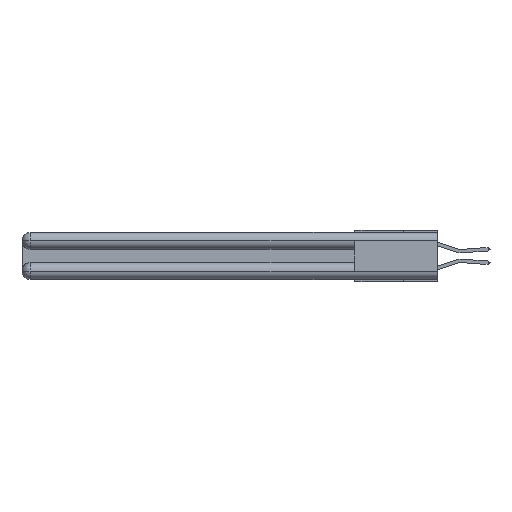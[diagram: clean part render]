
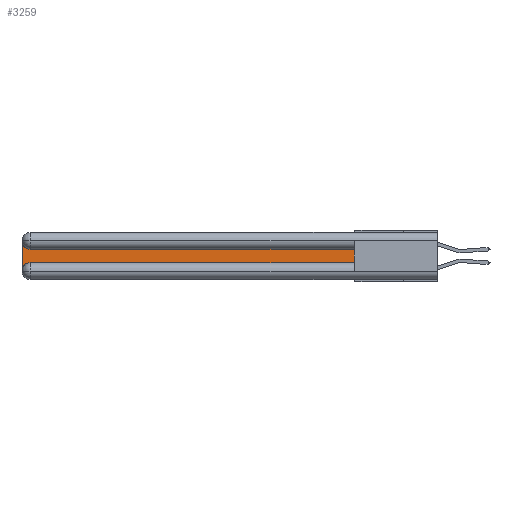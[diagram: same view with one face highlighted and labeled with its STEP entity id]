
A CAD part, left-side view. The second image highlights one B-rep face of the part: STEP entity #3259.
In plain terms, the highlighted planar face has unit normal (-1, 0, 0).
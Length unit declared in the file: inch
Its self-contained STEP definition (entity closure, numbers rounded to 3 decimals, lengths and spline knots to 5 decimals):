
#345 = CARTESIAN_POINT ( 'NONE',  ( 0.075, 2.94, -0.2775 ) ) ;
#422 = VECTOR ( 'NONE', #17137, 39.37008 ) ;
#693 = CARTESIAN_POINT ( 'NONE',  ( 0.075, 0.6, -0.1225 ) ) ;
#921 = AXIS2_PLACEMENT_3D ( 'NONE', #20512, #23227, #17745 ) ;
#1633 = CIRCLE ( 'NONE', #7621, 0.06 ) ;
#1658 = ORIENTED_EDGE ( 'NONE', *, *, #11270, .T. ) ;
#1872 = CARTESIAN_POINT ( 'NONE',  ( 0.075, 0.6, -0.1225 ) ) ;
#2462 = EDGE_CURVE ( 'NONE', #32187, #11492, #11005, .T. ) ;
#2471 = VERTEX_POINT ( 'NONE', #18239 ) ;
#2899 = DIRECTION ( 'NONE',  ( 1., 0., 0. ) ) ;
#3259 = ADVANCED_FACE ( 'NONE', ( #13729 ), #5594, .F. ) ;
#3362 = CARTESIAN_POINT ( 'NONE',  ( 0.075, 2.94, -0.2175 ) ) ;
#5594 = PLANE ( 'NONE',  #921 ) ;
#5992 = ORIENTED_EDGE ( 'NONE', *, *, #32218, .T. ) ;
#6529 = DIRECTION ( 'NONE',  ( 0., 0., -1. ) ) ;
#7053 = VECTOR ( 'NONE', #26360, 39.37008 ) ;
#7621 = AXIS2_PLACEMENT_3D ( 'NONE', #19111, #19005, #6529 ) ;
#8531 = CARTESIAN_POINT ( 'NONE',  ( 0.075, 3., -0.2775 ) ) ;
#8834 = ORIENTED_EDGE ( 'NONE', *, *, #2462, .T. ) ;
#9032 = EDGE_CURVE ( 'NONE', #11203, #17176, #18721, .T. ) ;
#9542 = CARTESIAN_POINT ( 'NONE',  ( 0.075, 0.6, -0.2175 ) ) ;
#10219 = ORIENTED_EDGE ( 'NONE', *, *, #11001, .T. ) ;
#11001 = EDGE_CURVE ( 'NONE', #17176, #32187, #1633, .T. ) ;
#11005 = LINE ( 'NONE', #31234, #12163 ) ;
#11203 = VERTEX_POINT ( 'NONE', #693 ) ;
#11270 = EDGE_CURVE ( 'NONE', #24827, #2471, #26851, .T. ) ;
#11492 = VERTEX_POINT ( 'NONE', #8531 ) ;
#12163 = VECTOR ( 'NONE', #16133, 39.37008 ) ;
#13073 = DIRECTION ( 'NONE',  ( 0., 0., -1. ) ) ;
#13291 = CARTESIAN_POINT ( 'NONE',  ( 0.075, 3., -0.0625 ) ) ;
#13729 = FACE_OUTER_BOUND ( 'NONE', #24518, .T. ) ;
#13787 = LINE ( 'NONE', #23938, #7053 ) ;
#14293 = CIRCLE ( 'NONE', #29495, 0.06 ) ;
#14594 = CARTESIAN_POINT ( 'NONE',  ( 0.075, 2.94, -0.1225 ) ) ;
#15156 = VECTOR ( 'NONE', #21952, 39.37008 ) ;
#16133 = DIRECTION ( 'NONE',  ( 0., 0., -1. ) ) ;
#17137 = DIRECTION ( 'NONE',  ( 0., -1., 0. ) ) ;
#17176 = VERTEX_POINT ( 'NONE', #14594 ) ;
#17745 = DIRECTION ( 'NONE',  ( 0., 0., -1. ) ) ;
#18239 = CARTESIAN_POINT ( 'NONE',  ( 0.075, 0.6, -0.2175 ) ) ;
#18721 = LINE ( 'NONE', #1872, #15156 ) ;
#19005 = DIRECTION ( 'NONE',  ( 1., 0., 0. ) ) ;
#19111 = CARTESIAN_POINT ( 'NONE',  ( 0.075, 2.94, -0.0625 ) ) ;
#19907 = ORIENTED_EDGE ( 'NONE', *, *, #27770, .T. ) ;
#20512 = CARTESIAN_POINT ( 'NONE',  ( 0.075, 3., -0.1225 ) ) ;
#21952 = DIRECTION ( 'NONE',  ( 0., 1., 0. ) ) ;
#23227 = DIRECTION ( 'NONE',  ( 1., 0., 0. ) ) ;
#23938 = CARTESIAN_POINT ( 'NONE',  ( 0.075, 0.6, -0.2175 ) ) ;
#24518 = EDGE_LOOP ( 'NONE', ( #30826, #10219, #8834, #5992, #1658, #19907 ) ) ;
#24827 = VERTEX_POINT ( 'NONE', #3362 ) ;
#26360 = DIRECTION ( 'NONE',  ( 0., 0., 1. ) ) ;
#26851 = LINE ( 'NONE', #9542, #422 ) ;
#27770 = EDGE_CURVE ( 'NONE', #2471, #11203, #13787, .T. ) ;
#29495 = AXIS2_PLACEMENT_3D ( 'NONE', #345, #2899, #13073 ) ;
#30826 = ORIENTED_EDGE ( 'NONE', *, *, #9032, .T. ) ;
#31234 = CARTESIAN_POINT ( 'NONE',  ( 0.075, 3., -0.2175 ) ) ;
#32187 = VERTEX_POINT ( 'NONE', #13291 ) ;
#32218 = EDGE_CURVE ( 'NONE', #11492, #24827, #14293, .T. ) ;
